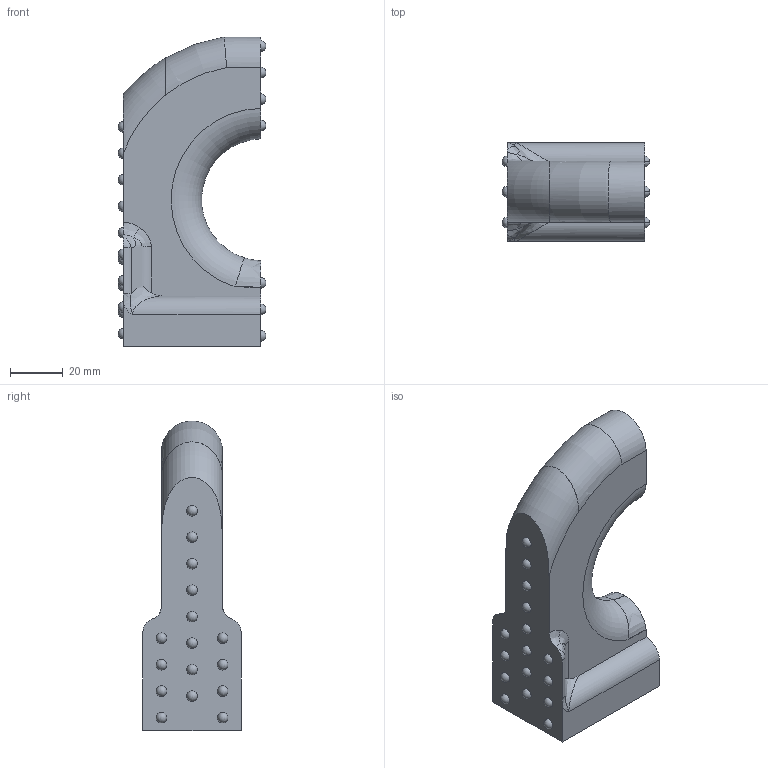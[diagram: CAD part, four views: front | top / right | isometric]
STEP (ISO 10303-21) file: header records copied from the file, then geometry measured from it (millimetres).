
FILE_DESCRIPTION (( 'STEP AP214' ), '1' );
FILE_NAME ('Charon_V3_Carbine_1.STEP', '2013-09-01T16:57:11', ( 'Asher' ), ( '' ), 'SwSTEP 2.0', 'SolidWorks 2013', '' );
FILE_SCHEMA (( 'AUTOMOTIVE_DESIGN' ));
Length unit declared in the file: inch
Products named in the file (1): Charon_V3_Carbine_1
Bounding box: 55.83 x 37.13 x 117.02 mm (x, y, z)
Volume: 121638.7 mm3; surface area: 19006 mm2
Topology: 1 solids, 1 shells, 90 faces, 297 edges, 180 vertices
Faces by surface type: sphere 49, bspline 16, plane 11, cylinder 10, torus 4
Entity records: 3819 total; most frequent: CARTESIAN_POINT 1783, DIRECTION 408, ORIENTED_EDGE 402, EDGE_CURVE 201, AXIS2_PLACEMENT_3D 187, VERTEX_POINT 149, EDGE_LOOP 126, CIRCLE 112
